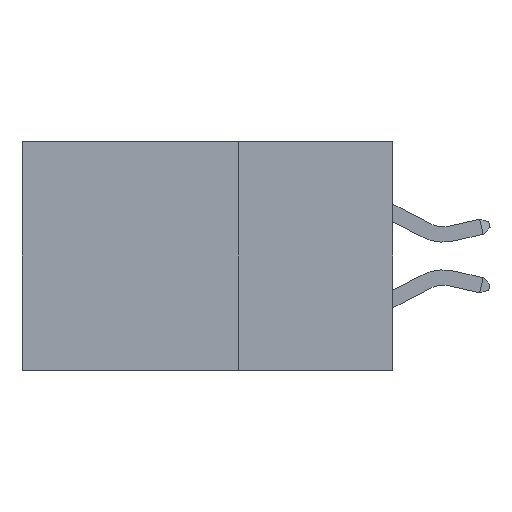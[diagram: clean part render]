
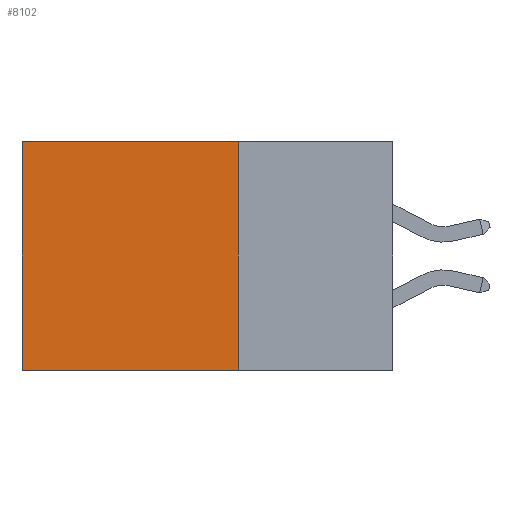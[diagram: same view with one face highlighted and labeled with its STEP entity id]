
A CAD part, left-side view. The second image highlights one B-rep face of the part: STEP entity #8102.
In plain terms, the highlighted planar face has unit normal (-1, 0, 0).
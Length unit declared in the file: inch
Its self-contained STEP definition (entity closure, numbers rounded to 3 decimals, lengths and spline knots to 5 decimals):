
#1081 = LINE ( 'NONE', #25260, #13012 ) ;
#1175 = DIRECTION ( 'NONE',  ( 0., 0., -1. ) ) ;
#1537 = LINE ( 'NONE', #3959, #9525 ) ;
#1548 = CARTESIAN_POINT ( 'NONE',  ( 0.2875, 0.25, 0. ) ) ;
#1738 = VERTEX_POINT ( 'NONE', #14874 ) ;
#3151 = DIRECTION ( 'NONE',  ( 0., 1., 0. ) ) ;
#3512 = CARTESIAN_POINT ( 'NONE',  ( 0.2875, 0.6, 0. ) ) ;
#3537 = CARTESIAN_POINT ( 'NONE',  ( 0.2875, 0.25, 0. ) ) ;
#3820 = FACE_OUTER_BOUND ( 'NONE', #4209, .T. ) ;
#3840 = LINE ( 'NONE', #1548, #12353 ) ;
#3959 = CARTESIAN_POINT ( 'NONE',  ( 0.2875, 0.25, -0.37 ) ) ;
#4209 = EDGE_LOOP ( 'NONE', ( #21894, #5783, #6628, #22586 ) ) ;
#5504 = CARTESIAN_POINT ( 'NONE',  ( 0.2875, 0.25, -0.37 ) ) ;
#5783 = ORIENTED_EDGE ( 'NONE', *, *, #9471, .F. ) ;
#6628 = ORIENTED_EDGE ( 'NONE', *, *, #27594, .F. ) ;
#7419 = DIRECTION ( 'NONE',  ( 0., 0., -1. ) ) ;
#7688 = CARTESIAN_POINT ( 'NONE',  ( 0.2875, 0.25, 0. ) ) ;
#8102 = ADVANCED_FACE ( 'NONE', ( #3820 ), #20951, .F. ) ;
#9471 = EDGE_CURVE ( 'NONE', #26130, #1738, #1537, .T. ) ;
#9525 = VECTOR ( 'NONE', #3151, 39.37008 ) ;
#11209 = AXIS2_PLACEMENT_3D ( 'NONE', #3537, #16621, #21376 ) ;
#12353 = VECTOR ( 'NONE', #14626, 39.37008 ) ;
#13012 = VECTOR ( 'NONE', #7419, 39.37008 ) ;
#14125 = LINE ( 'NONE', #24941, #27755 ) ;
#14626 = DIRECTION ( 'NONE',  ( 0., 1., 0. ) ) ;
#14874 = CARTESIAN_POINT ( 'NONE',  ( 0.2875, 0.6, -0.37 ) ) ;
#15895 = EDGE_CURVE ( 'NONE', #19339, #19352, #3840, .T. ) ;
#16621 = DIRECTION ( 'NONE',  ( 1., 0., 0. ) ) ;
#19339 = VERTEX_POINT ( 'NONE', #7688 ) ;
#19352 = VERTEX_POINT ( 'NONE', #3512 ) ;
#20951 = PLANE ( 'NONE',  #11209 ) ;
#21376 = DIRECTION ( 'NONE',  ( 0., 0., -1. ) ) ;
#21894 = ORIENTED_EDGE ( 'NONE', *, *, #27141, .T. ) ;
#22586 = ORIENTED_EDGE ( 'NONE', *, *, #15895, .T. ) ;
#24941 = CARTESIAN_POINT ( 'NONE',  ( 0.2875, 0.25, 0. ) ) ;
#25260 = CARTESIAN_POINT ( 'NONE',  ( 0.2875, 0.6, 0. ) ) ;
#26130 = VERTEX_POINT ( 'NONE', #5504 ) ;
#27141 = EDGE_CURVE ( 'NONE', #19352, #1738, #1081, .T. ) ;
#27594 = EDGE_CURVE ( 'NONE', #19339, #26130, #14125, .T. ) ;
#27755 = VECTOR ( 'NONE', #1175, 39.37008 ) ;
